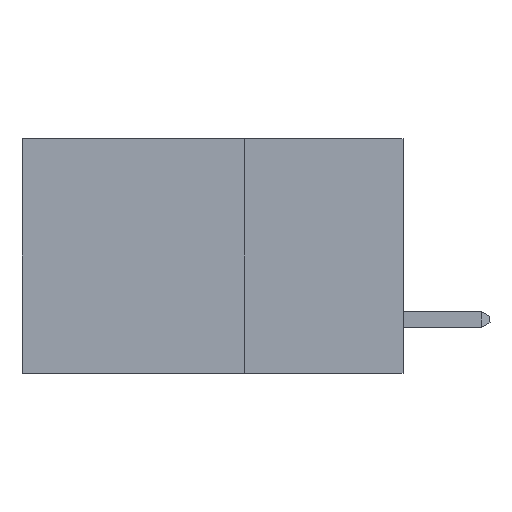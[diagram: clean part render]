
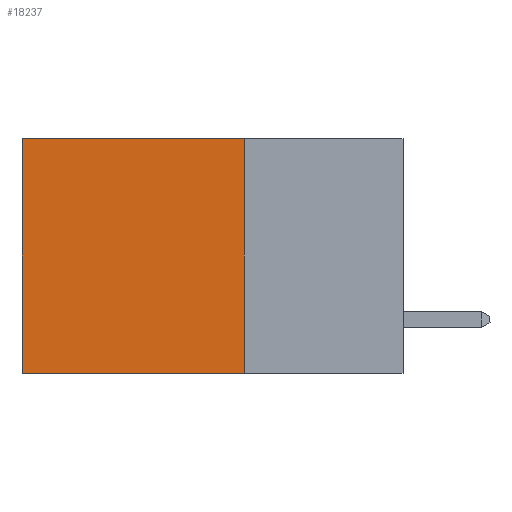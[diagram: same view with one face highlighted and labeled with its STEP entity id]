
A CAD part, left-side view. The second image highlights one B-rep face of the part: STEP entity #18237.
In plain terms, the highlighted planar face has unit normal (-1, 0, 0).
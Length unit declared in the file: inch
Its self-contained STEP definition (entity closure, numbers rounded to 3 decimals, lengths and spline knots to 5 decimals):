
#1273 = FACE_OUTER_BOUND ( 'NONE', #2138, .T. ) ;
#2138 = EDGE_LOOP ( 'NONE', ( #9796, #5186, #15199, #17629 ) ) ;
#2690 = VECTOR ( 'NONE', #6211, 39.37008 ) ;
#2771 = DIRECTION ( 'NONE',  ( 0., 1., 0. ) ) ;
#2975 = CARTESIAN_POINT ( 'NONE',  ( 0.2875, 0.25, 0. ) ) ;
#4134 = VERTEX_POINT ( 'NONE', #2975 ) ;
#4724 = EDGE_CURVE ( 'NONE', #19287, #8450, #8480, .T. ) ;
#5186 = ORIENTED_EDGE ( 'NONE', *, *, #4724, .F. ) ;
#6072 = VECTOR ( 'NONE', #10098, 39.37008 ) ;
#6211 = DIRECTION ( 'NONE',  ( 0., 0., -1. ) ) ;
#7434 = DIRECTION ( 'NONE',  ( 0., 0., -1. ) ) ;
#7766 = VERTEX_POINT ( 'NONE', #11887 ) ;
#7773 = CARTESIAN_POINT ( 'NONE',  ( 0.2875, 0.25, 0. ) ) ;
#7969 = VECTOR ( 'NONE', #8158, 39.37008 ) ;
#8158 = DIRECTION ( 'NONE',  ( 0., 1., 0. ) ) ;
#8450 = VERTEX_POINT ( 'NONE', #13612 ) ;
#8480 = LINE ( 'NONE', #18708, #7969 ) ;
#9796 = ORIENTED_EDGE ( 'NONE', *, *, #12588, .T. ) ;
#10098 = DIRECTION ( 'NONE',  ( 0., 0., -1. ) ) ;
#10503 = CARTESIAN_POINT ( 'NONE',  ( 0.2875, 0.25, 0. ) ) ;
#10555 = CARTESIAN_POINT ( 'NONE',  ( 0.2875, 0.25, 0. ) ) ;
#10964 = LINE ( 'NONE', #7773, #2690 ) ;
#11033 = AXIS2_PLACEMENT_3D ( 'NONE', #10503, #16522, #7434 ) ;
#11522 = CARTESIAN_POINT ( 'NONE',  ( 0.2875, 0.25, -0.37 ) ) ;
#11887 = CARTESIAN_POINT ( 'NONE',  ( 0.2875, 0.6, 0. ) ) ;
#12588 = EDGE_CURVE ( 'NONE', #7766, #8450, #14162, .T. ) ;
#13612 = CARTESIAN_POINT ( 'NONE',  ( 0.2875, 0.6, -0.37 ) ) ;
#14162 = LINE ( 'NONE', #16047, #6072 ) ;
#14402 = EDGE_CURVE ( 'NONE', #4134, #19287, #10964, .T. ) ;
#14609 = LINE ( 'NONE', #10555, #18148 ) ;
#14979 = PLANE ( 'NONE',  #11033 ) ;
#15199 = ORIENTED_EDGE ( 'NONE', *, *, #14402, .F. ) ;
#16047 = CARTESIAN_POINT ( 'NONE',  ( 0.2875, 0.6, 0. ) ) ;
#16522 = DIRECTION ( 'NONE',  ( 1., 0., 0. ) ) ;
#16932 = EDGE_CURVE ( 'NONE', #4134, #7766, #14609, .T. ) ;
#17629 = ORIENTED_EDGE ( 'NONE', *, *, #16932, .T. ) ;
#18148 = VECTOR ( 'NONE', #2771, 39.37008 ) ;
#18237 = ADVANCED_FACE ( 'NONE', ( #1273 ), #14979, .F. ) ;
#18708 = CARTESIAN_POINT ( 'NONE',  ( 0.2875, 0.25, -0.37 ) ) ;
#19287 = VERTEX_POINT ( 'NONE', #11522 ) ;
